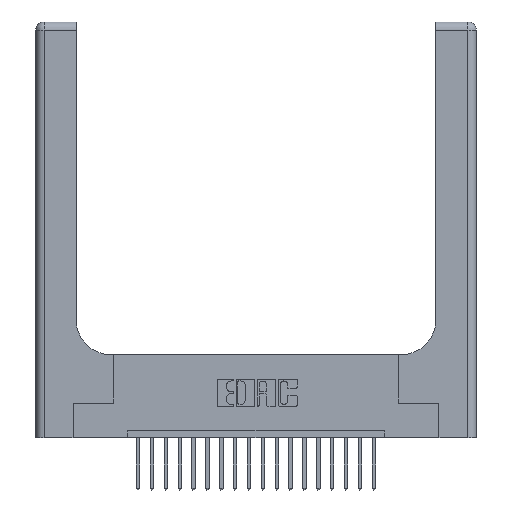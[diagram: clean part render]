
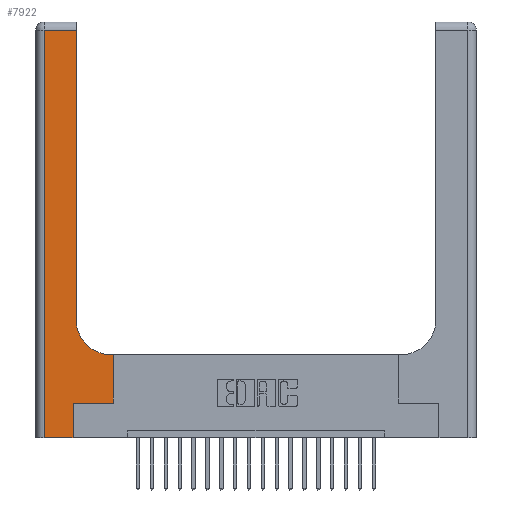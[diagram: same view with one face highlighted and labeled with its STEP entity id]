
A CAD part, top view. The second image highlights one B-rep face of the part: STEP entity #7922.
In plain terms, the highlighted planar face has unit normal (0, 0, 1).
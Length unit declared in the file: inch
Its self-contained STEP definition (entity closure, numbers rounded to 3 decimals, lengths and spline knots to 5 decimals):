
#178 = VECTOR ( 'NONE', #14043, 39.37008 ) ;
#259 = ORIENTED_EDGE ( 'NONE', *, *, #15437, .T. ) ;
#648 = EDGE_CURVE ( 'NONE', #685, #10528, #4131, .T. ) ;
#685 = VERTEX_POINT ( 'NONE', #12080 ) ;
#717 = ORIENTED_EDGE ( 'NONE', *, *, #3284, .T. ) ;
#1029 = DIRECTION ( 'NONE',  ( 0., 1., 0. ) ) ;
#1382 = CARTESIAN_POINT ( 'NONE',  ( 0.06, 0., 0.37 ) ) ;
#1755 = VERTEX_POINT ( 'NONE', #1382 ) ;
#1941 = CARTESIAN_POINT ( 'NONE',  ( 0.5585, 0.25, 0.37 ) ) ;
#2228 = AXIS2_PLACEMENT_3D ( 'NONE', #10185, #15150, #15074 ) ;
#2655 = DIRECTION ( 'NONE',  ( 1., 0., 0. ) ) ;
#2714 = DIRECTION ( 'NONE',  ( 0., -1., 0. ) ) ;
#2838 = CARTESIAN_POINT ( 'NONE',  ( 0.2915, 3., 0.37 ) ) ;
#3284 = EDGE_CURVE ( 'NONE', #1755, #15423, #4766, .T. ) ;
#3511 = EDGE_CURVE ( 'NONE', #18969, #15435, #9217, .T. ) ;
#4131 = LINE ( 'NONE', #2838, #7313 ) ;
#4766 = LINE ( 'NONE', #16001, #8707 ) ;
#5025 = ORIENTED_EDGE ( 'NONE', *, *, #3511, .T. ) ;
#5148 = CARTESIAN_POINT ( 'NONE',  ( 0.2915, 2.94, 0.37 ) ) ;
#5832 = VECTOR ( 'NONE', #17051, 39.37008 ) ;
#5925 = VECTOR ( 'NONE', #18901, 39.37008 ) ;
#6001 = DIRECTION ( 'NONE',  ( 0., 0., -1. ) ) ;
#6098 = ORIENTED_EDGE ( 'NONE', *, *, #19429, .T. ) ;
#6889 = ORIENTED_EDGE ( 'NONE', *, *, #18355, .T. ) ;
#7313 = VECTOR ( 'NONE', #1029, 39.37008 ) ;
#7922 = ADVANCED_FACE ( 'NONE', ( #18615 ), #10105, .F. ) ;
#8166 = EDGE_CURVE ( 'NONE', #12626, #1755, #18861, .T. ) ;
#8386 = AXIS2_PLACEMENT_3D ( 'NONE', #10862, #6001, #9303 ) ;
#8402 = VERTEX_POINT ( 'NONE', #14078 ) ;
#8707 = VECTOR ( 'NONE', #2655, 39.37008 ) ;
#9217 = LINE ( 'NONE', #13270, #11606 ) ;
#9303 = DIRECTION ( 'NONE',  ( 1., 0., 0. ) ) ;
#9735 = VERTEX_POINT ( 'NONE', #18528 ) ;
#9774 = LINE ( 'NONE', #18955, #178 ) ;
#10028 = DIRECTION ( 'NONE',  ( 1., 0., 0. ) ) ;
#10105 = PLANE ( 'NONE',  #2228 ) ;
#10185 = CARTESIAN_POINT ( 'NONE',  ( 0., 3., 0.37 ) ) ;
#10322 = CARTESIAN_POINT ( 'NONE',  ( 0.2915, 0.6, 0.37 ) ) ;
#10528 = VERTEX_POINT ( 'NONE', #5148 ) ;
#10862 = CARTESIAN_POINT ( 'NONE',  ( 0.5415, 0.85, 0.37 ) ) ;
#10999 = ORIENTED_EDGE ( 'NONE', *, *, #8166, .T. ) ;
#11606 = VECTOR ( 'NONE', #10028, 39.37008 ) ;
#12058 = CARTESIAN_POINT ( 'NONE',  ( 0., 2.94, 0.37 ) ) ;
#12078 = DIRECTION ( 'NONE',  ( -1., 0., 0. ) ) ;
#12080 = CARTESIAN_POINT ( 'NONE',  ( 0.2915, 0.85, 0.37 ) ) ;
#12626 = VERTEX_POINT ( 'NONE', #20872 ) ;
#13270 = CARTESIAN_POINT ( 'NONE',  ( 0.269, 0.25, 0.37 ) ) ;
#13795 = VECTOR ( 'NONE', #2714, 39.37008 ) ;
#13861 = EDGE_LOOP ( 'NONE', ( #16126, #21579, #10999, #717, #6889, #5025, #259, #6098, #17923 ) ) ;
#14043 = DIRECTION ( 'NONE',  ( 0., 1., 0. ) ) ;
#14078 = CARTESIAN_POINT ( 'NONE',  ( 0.5415, 0.6, 0.37 ) ) ;
#15074 = DIRECTION ( 'NONE',  ( -1., 0., 0. ) ) ;
#15150 = DIRECTION ( 'NONE',  ( 0., 0., -1. ) ) ;
#15423 = VERTEX_POINT ( 'NONE', #18965 ) ;
#15435 = VERTEX_POINT ( 'NONE', #1941 ) ;
#15437 = EDGE_CURVE ( 'NONE', #15435, #9735, #19428, .T. ) ;
#15593 = CARTESIAN_POINT ( 'NONE',  ( 0.269, 0.25, 0.37 ) ) ;
#16001 = CARTESIAN_POINT ( 'NONE',  ( 0., 0., 0.37 ) ) ;
#16126 = ORIENTED_EDGE ( 'NONE', *, *, #648, .T. ) ;
#16892 = VECTOR ( 'NONE', #12078, 39.37008 ) ;
#17051 = DIRECTION ( 'NONE',  ( -1., 0., 0. ) ) ;
#17286 = CARTESIAN_POINT ( 'NONE',  ( 0.5585, 0.25, 0.37 ) ) ;
#17738 = LINE ( 'NONE', #12058, #5832 ) ;
#17923 = ORIENTED_EDGE ( 'NONE', *, *, #21261, .T. ) ;
#18269 = EDGE_CURVE ( 'NONE', #10528, #12626, #17738, .T. ) ;
#18355 = EDGE_CURVE ( 'NONE', #15423, #18969, #9774, .T. ) ;
#18528 = CARTESIAN_POINT ( 'NONE',  ( 0.5585, 0.6, 0.37 ) ) ;
#18615 = FACE_OUTER_BOUND ( 'NONE', #13861, .T. ) ;
#18861 = LINE ( 'NONE', #19617, #13795 ) ;
#18901 = DIRECTION ( 'NONE',  ( 0., 1., 0. ) ) ;
#18955 = CARTESIAN_POINT ( 'NONE',  ( 0.269, 0., 0.37 ) ) ;
#18965 = CARTESIAN_POINT ( 'NONE',  ( 0.269, 0., 0.37 ) ) ;
#18969 = VERTEX_POINT ( 'NONE', #15593 ) ;
#19002 = LINE ( 'NONE', #10322, #16892 ) ;
#19428 = LINE ( 'NONE', #17286, #5925 ) ;
#19429 = EDGE_CURVE ( 'NONE', #9735, #8402, #19002, .T. ) ;
#19617 = CARTESIAN_POINT ( 'NONE',  ( 0.06, 3., 0.37 ) ) ;
#20491 = CIRCLE ( 'NONE', #8386, 0.25 ) ;
#20872 = CARTESIAN_POINT ( 'NONE',  ( 0.06, 2.94, 0.37 ) ) ;
#21261 = EDGE_CURVE ( 'NONE', #8402, #685, #20491, .T. ) ;
#21579 = ORIENTED_EDGE ( 'NONE', *, *, #18269, .T. ) ;
